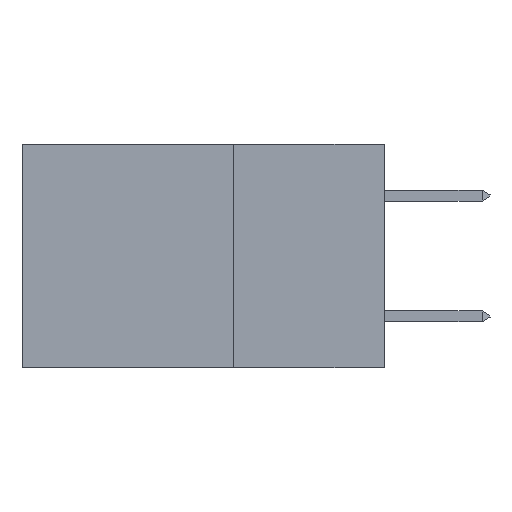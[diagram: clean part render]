
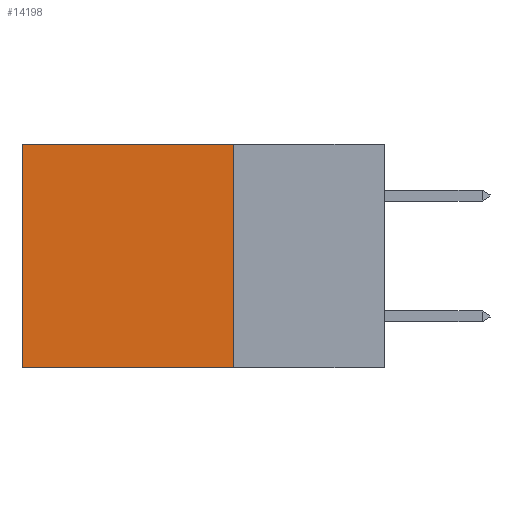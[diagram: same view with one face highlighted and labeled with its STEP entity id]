
A CAD part, left-side view. The second image highlights one B-rep face of the part: STEP entity #14198.
In plain terms, the highlighted planar face has unit normal (-1, 0, 0).
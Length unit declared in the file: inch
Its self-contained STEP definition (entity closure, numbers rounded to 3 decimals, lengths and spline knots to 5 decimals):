
#356 = AXIS2_PLACEMENT_3D ( 'NONE', #7639, #13578, #1699 ) ;
#1614 = EDGE_CURVE ( 'NONE', #17744, #11382, #9807, .T. ) ;
#1699 = DIRECTION ( 'NONE',  ( 0., 0., -1. ) ) ;
#1856 = CARTESIAN_POINT ( 'NONE',  ( 0.2875, 0.25, -0.37 ) ) ;
#2557 = VECTOR ( 'NONE', #22495, 39.37008 ) ;
#3071 = CARTESIAN_POINT ( 'NONE',  ( 0.2875, 0.25, -0.37 ) ) ;
#4644 = CARTESIAN_POINT ( 'NONE',  ( 0.2875, 0.6, -0.37 ) ) ;
#5612 = DIRECTION ( 'NONE',  ( 0., 0., -1. ) ) ;
#7279 = ORIENTED_EDGE ( 'NONE', *, *, #15419, .T. ) ;
#7436 = ORIENTED_EDGE ( 'NONE', *, *, #20814, .T. ) ;
#7639 = CARTESIAN_POINT ( 'NONE',  ( 0.2875, 0.25, 0. ) ) ;
#8682 = LINE ( 'NONE', #17287, #23388 ) ;
#9308 = CARTESIAN_POINT ( 'NONE',  ( 0.2875, 0.25, 0. ) ) ;
#9807 = LINE ( 'NONE', #9308, #19449 ) ;
#10298 = VERTEX_POINT ( 'NONE', #4644 ) ;
#11019 = CARTESIAN_POINT ( 'NONE',  ( 0.2875, 0.25, 0. ) ) ;
#11382 = VERTEX_POINT ( 'NONE', #3071 ) ;
#11604 = PLANE ( 'NONE',  #356 ) ;
#11647 = EDGE_LOOP ( 'NONE', ( #7279, #18364, #25088, #7436 ) ) ;
#12109 = FACE_OUTER_BOUND ( 'NONE', #11647, .T. ) ;
#13412 = VECTOR ( 'NONE', #13729, 39.37008 ) ;
#13578 = DIRECTION ( 'NONE',  ( 1., 0., 0. ) ) ;
#13729 = DIRECTION ( 'NONE',  ( 0., 1., 0. ) ) ;
#14198 = ADVANCED_FACE ( 'NONE', ( #12109 ), #11604, .F. ) ;
#15171 = CARTESIAN_POINT ( 'NONE',  ( 0.2875, 0.6, 0. ) ) ;
#15419 = EDGE_CURVE ( 'NONE', #16029, #10298, #8682, .T. ) ;
#16029 = VERTEX_POINT ( 'NONE', #15171 ) ;
#17287 = CARTESIAN_POINT ( 'NONE',  ( 0.2875, 0.6, 0. ) ) ;
#17744 = VERTEX_POINT ( 'NONE', #24434 ) ;
#18364 = ORIENTED_EDGE ( 'NONE', *, *, #21050, .F. ) ;
#18783 = LINE ( 'NONE', #11019, #2557 ) ;
#19449 = VECTOR ( 'NONE', #23059, 39.37008 ) ;
#20814 = EDGE_CURVE ( 'NONE', #17744, #16029, #18783, .T. ) ;
#21050 = EDGE_CURVE ( 'NONE', #11382, #10298, #22947, .T. ) ;
#22495 = DIRECTION ( 'NONE',  ( 0., 1., 0. ) ) ;
#22947 = LINE ( 'NONE', #1856, #13412 ) ;
#23059 = DIRECTION ( 'NONE',  ( 0., 0., -1. ) ) ;
#23388 = VECTOR ( 'NONE', #5612, 39.37008 ) ;
#24434 = CARTESIAN_POINT ( 'NONE',  ( 0.2875, 0.25, 0. ) ) ;
#25088 = ORIENTED_EDGE ( 'NONE', *, *, #1614, .F. ) ;
